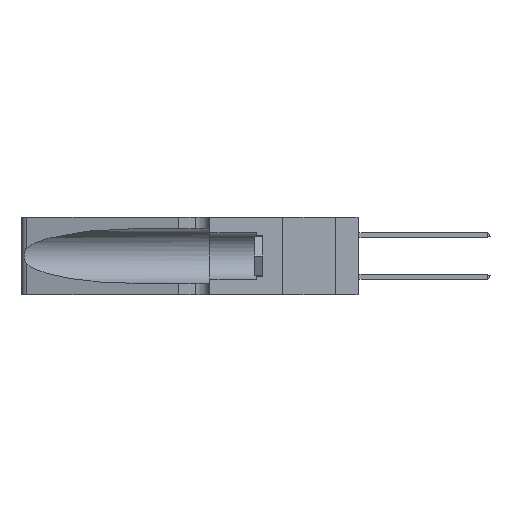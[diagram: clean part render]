
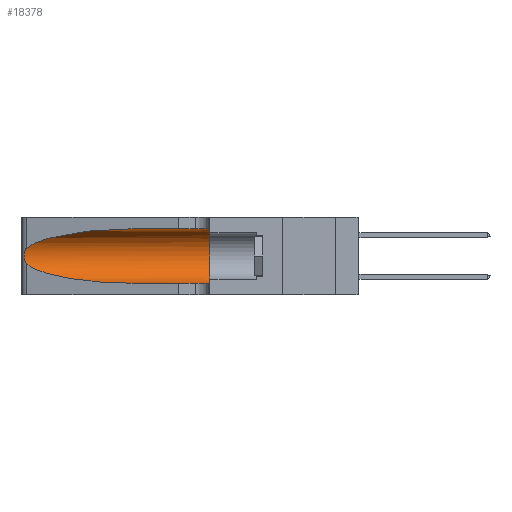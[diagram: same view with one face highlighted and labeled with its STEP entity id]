
A CAD part, left-side view. The second image highlights one B-rep face of the part: STEP entity #18378.
In plain terms, the highlighted cylindrical face has radius 3.308 mm (diameter 6.617 mm), a partial arc.
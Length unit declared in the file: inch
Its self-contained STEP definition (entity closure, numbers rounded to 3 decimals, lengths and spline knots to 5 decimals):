
#115 = CARTESIAN_POINT ( 'NONE',  ( 0.26075, 1.23896, 0.178 ) ) ;
#377 = DIRECTION ( 'NONE',  ( 0., 0., 1. ) ) ;
#416 = VERTEX_POINT ( 'NONE', #5994 ) ;
#483 = VERTEX_POINT ( 'NONE', #15206 ) ;
#858 = CYLINDRICAL_SURFACE ( 'NONE', #10457, 0.13025 ) ;
#1028 = AXIS2_PLACEMENT_3D ( 'NONE', #22180, #11552, #377 ) ;
#1167 = CARTESIAN_POINT ( 'NONE',  ( 0.25487, 1.22718, 0.22369 ) ) ;
#1270 = ORIENTED_EDGE ( 'NONE', *, *, #9755, .F. ) ;
#1416 = CARTESIAN_POINT ( 'NONE',  ( 0.1305, 0.35, 0.31525 ) ) ;
#2030 = CARTESIAN_POINT ( 'NONE',  ( 0.25856, 1.23593, 0.16098 ) ) ;
#2338 = VERTEX_POINT ( 'NONE', #10320 ) ;
#3622 = CARTESIAN_POINT ( 'NONE',  ( 0.18966, 0.96281, 0.31525 ) ) ;
#3647 = CARTESIAN_POINT ( 'NONE',  ( 0.1305, 1.61858, 0.185 ) ) ;
#3745 = CARTESIAN_POINT ( 'NONE',  ( 0.1305, 1.61858, 0.05475 ) ) ;
#3930 = CARTESIAN_POINT ( 'NONE',  ( 0.25639, 1.23186, 0.15144 ) ) ;
#4255 = CARTESIAN_POINT ( 'NONE',  ( 0.25487, 1.22718, 0.14631 ) ) ;
#4742 =( BOUNDED_CURVE ( )  B_SPLINE_CURVE ( 3, ( #23518, #3622, #18269, #1167 ),
 .UNSPECIFIED., .F., .F. ) 
 B_SPLINE_CURVE_WITH_KNOTS ( ( 4, 4 ),
 ( 1.5708, 2.84003 ),
 .UNSPECIFIED. ) 
 CURVE ( )  GEOMETRIC_REPRESENTATION_ITEM ( )  RATIONAL_B_SPLINE_CURVE ( ( 1., 0.87, 0.87, 1. ) ) 
 REPRESENTATION_ITEM ( '' )  );
#5772 = CARTESIAN_POINT ( 'NONE',  ( 0.25487, 1.22718, 0.14631 ) ) ;
#5994 = CARTESIAN_POINT ( 'NONE',  ( 0.1305, 0.72297, 0.05475 ) ) ;
#6117 = CARTESIAN_POINT ( 'NONE',  ( 0.18966, 0.96281, 0.05475 ) ) ;
#6339 = CARTESIAN_POINT ( 'NONE',  ( 0.1305, 1.61858, 0.31525 ) ) ;
#6482 = VERTEX_POINT ( 'NONE', #1416 ) ;
#7120 = ORIENTED_EDGE ( 'NONE', *, *, #7489, .T. ) ;
#7217 = DIRECTION ( 'NONE',  ( 0., -1., 0. ) ) ;
#7489 = EDGE_CURVE ( 'NONE', #17858, #416, #13310, .T. ) ;
#7598 = CARTESIAN_POINT ( 'NONE',  ( 0.25639, 1.23184, 0.21858 ) ) ;
#7727 = ORIENTED_EDGE ( 'NONE', *, *, #10064, .T. ) ;
#7756 = CARTESIAN_POINT ( 'NONE',  ( 0.25487, 1.22718, 0.14631 ) ) ;
#9010 = LINE ( 'NONE', #6339, #13296 ) ;
#9224 = CIRCLE ( 'NONE', #1028, 0.13025 ) ;
#9454 = CARTESIAN_POINT ( 'NONE',  ( 0.25854, 1.2359, 0.20912 ) ) ;
#9755 = EDGE_CURVE ( 'NONE', #2338, #6482, #9010, .T. ) ;
#10064 = EDGE_CURVE ( 'NONE', #416, #483, #17200, .T. ) ;
#10320 = CARTESIAN_POINT ( 'NONE',  ( 0.1305, 0.72297, 0.31525 ) ) ;
#10457 = AXIS2_PLACEMENT_3D ( 'NONE', #3647, #7217, #14643 ) ;
#11302 = CARTESIAN_POINT ( 'NONE',  ( 0.26075, 1.23896, 0.19203 ) ) ;
#11552 = DIRECTION ( 'NONE',  ( 0., 1., 0. ) ) ;
#13129 = CARTESIAN_POINT ( 'NONE',  ( 0.26017, 1.23833, 0.17102 ) ) ;
#13296 = VECTOR ( 'NONE', #15473, 39.37008 ) ;
#13310 =( BOUNDED_CURVE ( )  B_SPLINE_CURVE ( 3, ( #4255, #17049, #6117, #18815 ),
 .UNSPECIFIED., .F., .T. ) 
 B_SPLINE_CURVE_WITH_KNOTS ( ( 4, 4 ),
 ( 3.44316, 4.71239 ),
 .UNSPECIFIED. ) 
 CURVE ( )  GEOMETRIC_REPRESENTATION_ITEM ( )  RATIONAL_B_SPLINE_CURVE ( ( 1., 0.87, 0.87, 1. ) ) 
 REPRESENTATION_ITEM ( '' )  );
#13970 = EDGE_CURVE ( 'NONE', #2338, #18936, #4742, .T. ) ;
#14643 = DIRECTION ( 'NONE',  ( 0., 0., -1. ) ) ;
#14917 = EDGE_CURVE ( 'NONE', #18936, #17858, #19841, .T. ) ;
#14921 = CARTESIAN_POINT ( 'NONE',  ( 0.25789, 1.23486, 0.15765 ) ) ;
#14978 = EDGE_CURVE ( 'NONE', #6482, #483, #9224, .T. ) ;
#15206 = CARTESIAN_POINT ( 'NONE',  ( 0.1305, 0.35, 0.05475 ) ) ;
#15473 = DIRECTION ( 'NONE',  ( 0., -1., 0. ) ) ;
#15576 = FACE_OUTER_BOUND ( 'NONE', #20060, .T. ) ;
#15685 = ORIENTED_EDGE ( 'NONE', *, *, #13970, .T. ) ;
#16196 = CARTESIAN_POINT ( 'NONE',  ( 0.25487, 1.22718, 0.22369 ) ) ;
#16644 = CARTESIAN_POINT ( 'NONE',  ( 0.25487, 1.22718, 0.22369 ) ) ;
#16730 = CARTESIAN_POINT ( 'NONE',  ( 0.25555, 1.22993, 0.14849 ) ) ;
#17049 = CARTESIAN_POINT ( 'NONE',  ( 0.2373, 1.15595, 0.08982 ) ) ;
#17200 = LINE ( 'NONE', #3745, #21303 ) ;
#17858 = VERTEX_POINT ( 'NONE', #7756 ) ;
#17908 = ORIENTED_EDGE ( 'NONE', *, *, #14978, .F. ) ;
#18269 = CARTESIAN_POINT ( 'NONE',  ( 0.2373, 1.15595, 0.28018 ) ) ;
#18324 = DIRECTION ( 'NONE',  ( 0., -1., 0. ) ) ;
#18378 = ADVANCED_FACE ( 'NONE', ( #15576 ), #858, .F. ) ;
#18416 = CARTESIAN_POINT ( 'NONE',  ( 0.25555, 1.22994, 0.2215 ) ) ;
#18815 = CARTESIAN_POINT ( 'NONE',  ( 0.1305, 0.72297, 0.05475 ) ) ;
#18936 = VERTEX_POINT ( 'NONE', #16196 ) ;
#19841 = B_SPLINE_CURVE_WITH_KNOTS ( 'NONE', 3,
 ( #16644, #18416, #7598, #20169, #9454, #21950, #11302, #115, #13129, #2030, #14921, #3930, #16730, #5772 ),
 .UNSPECIFIED., .F., .F.,
 ( 4, 2, 2, 2, 2, 2, 4 ),
 ( 0., 0.00027, 0.00053, 0.00107, 0.0016, 0.00187, 0.00214 ),
 .UNSPECIFIED. ) ;
#20060 = EDGE_LOOP ( 'NONE', ( #15685, #20368, #7120, #7727, #17908, #1270 ) ) ;
#20169 = CARTESIAN_POINT ( 'NONE',  ( 0.25787, 1.23484, 0.2124 ) ) ;
#20368 = ORIENTED_EDGE ( 'NONE', *, *, #14917, .T. ) ;
#21303 = VECTOR ( 'NONE', #18324, 39.37008 ) ;
#21950 = CARTESIAN_POINT ( 'NONE',  ( 0.26018, 1.23835, 0.19895 ) ) ;
#22180 = CARTESIAN_POINT ( 'NONE',  ( 0.1305, 0.35, 0.185 ) ) ;
#23518 = CARTESIAN_POINT ( 'NONE',  ( 0.1305, 0.72297, 0.31525 ) ) ;
